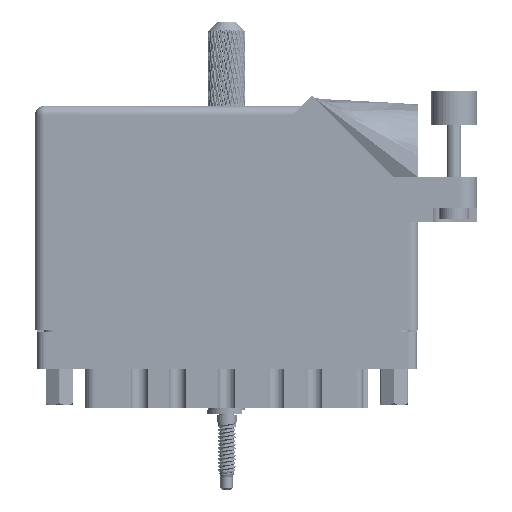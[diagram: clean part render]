
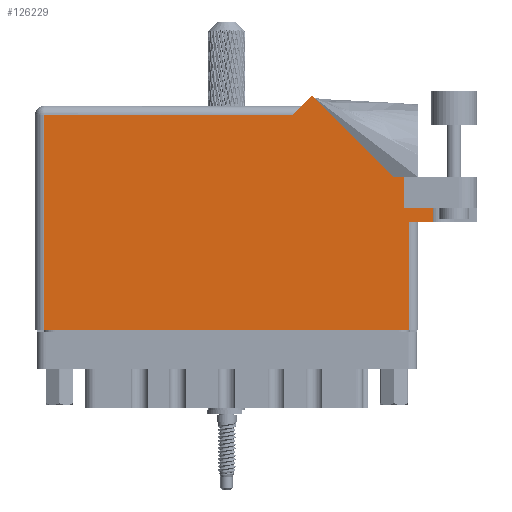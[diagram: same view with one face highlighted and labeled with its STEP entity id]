
A CAD part, front view. The second image highlights one B-rep face of the part: STEP entity #126229.
In plain terms, the highlighted face is planar.
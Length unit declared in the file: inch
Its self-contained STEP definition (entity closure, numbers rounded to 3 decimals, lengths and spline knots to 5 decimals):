
#1104 = DIRECTION ( 'NONE',  ( -0.707, 0.707, 0. ) ) ;
#1584 = EDGE_CURVE ( 'NONE', #11302, #114797, #31526, .T. ) ;
#2825 = CARTESIAN_POINT ( 'NONE',  ( 1.88971, 1.60071, 0. ) ) ;
#4908 = EDGE_CURVE ( 'NONE', #11469, #11302, #97870, .T. ) ;
#9393 = VERTEX_POINT ( 'NONE', #111923 ) ;
#11302 = VERTEX_POINT ( 'NONE', #2825 ) ;
#11469 = VERTEX_POINT ( 'NONE', #59683 ) ;
#14624 = EDGE_CURVE ( 'NONE', #64015, #28244, #108464, .T. ) ;
#17697 = LINE ( 'NONE', #56682, #65493 ) ;
#19498 = VECTOR ( 'NONE', #22870, 39.37008 ) ;
#20959 = DIRECTION ( 'NONE',  ( 0., 0., -1. ) ) ;
#21260 = VECTOR ( 'NONE', #105465, 39.37008 ) ;
#21847 = LINE ( 'NONE', #60803, #47026 ) ;
#22410 = EDGE_CURVE ( 'NONE', #9393, #98703, #85296, .T. ) ;
#22870 = DIRECTION ( 'NONE',  ( -1., 0., 0. ) ) ;
#23193 = VECTOR ( 'NONE', #88338, 39.37008 ) ;
#23771 = ORIENTED_EDGE ( 'NONE', *, *, #97544, .T. ) ;
#28244 = VERTEX_POINT ( 'NONE', #33555 ) ;
#29761 = LINE ( 'NONE', #111606, #44106 ) ;
#31351 = DIRECTION ( 'NONE',  ( -1., 0., 0. ) ) ;
#31496 = VECTOR ( 'NONE', #53687, 39.37008 ) ;
#31526 = LINE ( 'NONE', #81530, #123528 ) ;
#32002 = LINE ( 'NONE', #63748, #19498 ) ;
#33507 = ORIENTED_EDGE ( 'NONE', *, *, #36183, .F. ) ;
#33555 = CARTESIAN_POINT ( 'NONE',  ( 2.512, 1.044, 0. ) ) ;
#36183 = EDGE_CURVE ( 'NONE', #53832, #90598, #17697, .T. ) ;
#37753 = CARTESIAN_POINT ( 'NONE',  ( 2.55, 0., 0. ) ) ;
#43184 = EDGE_CURVE ( 'NONE', #64015, #53832, #54667, .T. ) ;
#43553 = CARTESIAN_POINT ( 'NONE',  ( 2.7135, 0.831, 0. ) ) ;
#44106 = VECTOR ( 'NONE', #118749, 39.37008 ) ;
#47026 = VECTOR ( 'NONE', #110866, 39.37008 ) ;
#51370 = ORIENTED_EDGE ( 'NONE', *, *, #106106, .T. ) ;
#53386 = DIRECTION ( 'NONE',  ( 1., 0., 0. ) ) ;
#53687 = DIRECTION ( 'NONE',  ( 1., 0., 0. ) ) ;
#53832 = VERTEX_POINT ( 'NONE', #43553 ) ;
#54667 = LINE ( 'NONE', #72868, #125212 ) ;
#54753 = LINE ( 'NONE', #72322, #75072 ) ;
#56682 = CARTESIAN_POINT ( 'NONE',  ( 2.7135, 1.16177, 0. ) ) ;
#57308 = DIRECTION ( 'NONE',  ( 0., -1., 0. ) ) ;
#59683 = CARTESIAN_POINT ( 'NONE',  ( 2.44642, 1.044, 0. ) ) ;
#60803 = CARTESIAN_POINT ( 'NONE',  ( 0., 1.468, 0. ) ) ;
#63748 = CARTESIAN_POINT ( 'NONE',  ( 3.012, 1.044, 0. ) ) ;
#64015 = VERTEX_POINT ( 'NONE', #126316 ) ;
#65493 = VECTOR ( 'NONE', #57308, 39.37008 ) ;
#67355 = ORIENTED_EDGE ( 'NONE', *, *, #1584, .T. ) ;
#68932 = ORIENTED_EDGE ( 'NONE', *, *, #43184, .F. ) ;
#72322 = CARTESIAN_POINT ( 'NONE',  ( 2.55, 0.737, 0. ) ) ;
#72868 = CARTESIAN_POINT ( 'NONE',  ( 2.512, 0.831, 0. ) ) ;
#73623 = DIRECTION ( 'NONE',  ( 0., 1., 0. ) ) ;
#74410 = VERTEX_POINT ( 'NONE', #110592 ) ;
#74870 = ORIENTED_EDGE ( 'NONE', *, *, #114295, .T. ) ;
#75022 = ORIENTED_EDGE ( 'NONE', *, *, #22410, .T. ) ;
#75072 = VECTOR ( 'NONE', #73623, 39.37008 ) ;
#80090 = FACE_OUTER_BOUND ( 'NONE', #87733, .T. ) ;
#81530 = CARTESIAN_POINT ( 'NONE',  ( 1.819, 1.53, 0. ) ) ;
#81783 = ORIENTED_EDGE ( 'NONE', *, *, #4908, .T. ) ;
#84846 = LINE ( 'NONE', #124483, #31496 ) ;
#85296 = LINE ( 'NONE', #124937, #21260 ) ;
#87733 = EDGE_LOOP ( 'NONE', ( #23771, #123561, #88493, #33507, #68932, #92999, #51370, #81783, #67355, #74870, #75022 ) ) ;
#88338 = DIRECTION ( 'NONE',  ( 0., 1., 0. ) ) ;
#88433 = EDGE_CURVE ( 'NONE', #110229, #74410, #54753, .T. ) ;
#88493 = ORIENTED_EDGE ( 'NONE', *, *, #100451, .T. ) ;
#90598 = VERTEX_POINT ( 'NONE', #118595 ) ;
#92999 = ORIENTED_EDGE ( 'NONE', *, *, #14624, .T. ) ;
#97544 = EDGE_CURVE ( 'NONE', #98703, #110229, #84846, .T. ) ;
#97870 = LINE ( 'NONE', #99818, #99013 ) ;
#98074 = CARTESIAN_POINT ( 'NONE',  ( 2.512, 0.831, 0. ) ) ;
#98703 = VERTEX_POINT ( 'NONE', #114278 ) ;
#99013 = VECTOR ( 'NONE', #1104, 39.37008 ) ;
#99818 = CARTESIAN_POINT ( 'NONE',  ( 2.44642, 1.044, 0. ) ) ;
#100451 = EDGE_CURVE ( 'NONE', #74410, #90598, #29761, .T. ) ;
#105465 = DIRECTION ( 'NONE',  ( 0., -1., 0. ) ) ;
#106106 = EDGE_CURVE ( 'NONE', #28244, #11469, #32002, .T. ) ;
#108464 = LINE ( 'NONE', #98074, #23193 ) ;
#109971 = CARTESIAN_POINT ( 'NONE',  ( 0., 1.53, 0. ) ) ;
#110229 = VERTEX_POINT ( 'NONE', #37753 ) ;
#110592 = CARTESIAN_POINT ( 'NONE',  ( 2.55, 0.737, 0. ) ) ;
#110866 = DIRECTION ( 'NONE',  ( -1., 0., 0. ) ) ;
#111436 = DIRECTION ( 'NONE',  ( -0.707, -0.707, 0. ) ) ;
#111606 = CARTESIAN_POINT ( 'NONE',  ( 2.612, 0.737, 0. ) ) ;
#111923 = CARTESIAN_POINT ( 'NONE',  ( 0.062, 1.468, 0. ) ) ;
#114278 = CARTESIAN_POINT ( 'NONE',  ( 0.062, 0., 0. ) ) ;
#114295 = EDGE_CURVE ( 'NONE', #114797, #9393, #21847, .T. ) ;
#114797 = VERTEX_POINT ( 'NONE', #127457 ) ;
#118595 = CARTESIAN_POINT ( 'NONE',  ( 2.7135, 0.737, 0. ) ) ;
#118749 = DIRECTION ( 'NONE',  ( 1., 0., 0. ) ) ;
#119721 = PLANE ( 'NONE',  #120343 ) ;
#120343 = AXIS2_PLACEMENT_3D ( 'NONE', #109971, #20959, #31351 ) ;
#123528 = VECTOR ( 'NONE', #111436, 39.37008 ) ;
#123561 = ORIENTED_EDGE ( 'NONE', *, *, #88433, .T. ) ;
#124483 = CARTESIAN_POINT ( 'NONE',  ( 0., 0., 0. ) ) ;
#124937 = CARTESIAN_POINT ( 'NONE',  ( 0.062, 0., 0. ) ) ;
#125212 = VECTOR ( 'NONE', #53386, 39.37008 ) ;
#126229 = ADVANCED_FACE ( 'NONE', ( #80090 ), #119721, .F. ) ;
#126316 = CARTESIAN_POINT ( 'NONE',  ( 2.512, 0.831, 0. ) ) ;
#127457 = CARTESIAN_POINT ( 'NONE',  ( 1.757, 1.468, 0. ) ) ;
